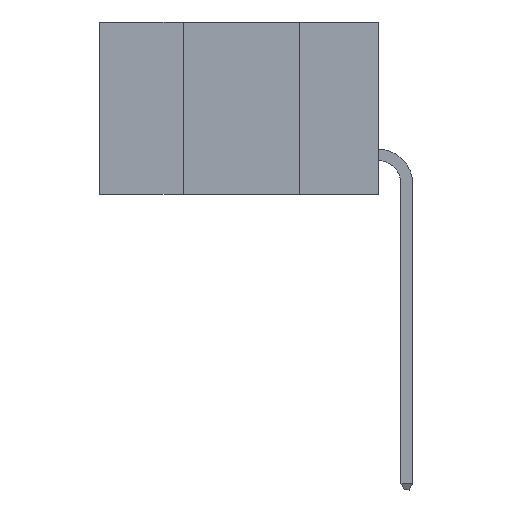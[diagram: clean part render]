
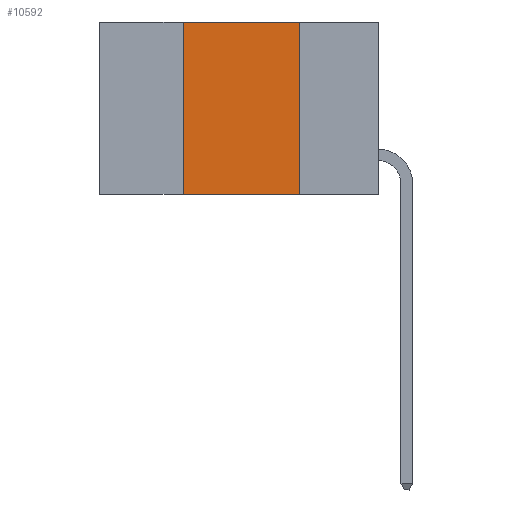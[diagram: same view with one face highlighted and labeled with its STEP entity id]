
A CAD part, left-side view. The second image highlights one B-rep face of the part: STEP entity #10592.
In plain terms, the highlighted planar face has unit normal (-1, 0, 0).
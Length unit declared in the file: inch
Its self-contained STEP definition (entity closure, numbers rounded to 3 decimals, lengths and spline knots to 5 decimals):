
#473 = CARTESIAN_POINT ( 'NONE',  ( 0., 0.42, 0. ) ) ;
#482 = CARTESIAN_POINT ( 'NONE',  ( 0., 0.17, -0.37 ) ) ;
#729 = VERTEX_POINT ( 'NONE', #4284 ) ;
#1281 = EDGE_CURVE ( 'NONE', #11646, #4821, #4223, .T. ) ;
#1575 = ORIENTED_EDGE ( 'NONE', *, *, #9898, .F. ) ;
#1997 = CARTESIAN_POINT ( 'NONE',  ( 0., 0.42, -0.37 ) ) ;
#2478 = LINE ( 'NONE', #9122, #4818 ) ;
#2542 = CARTESIAN_POINT ( 'NONE',  ( 0., 0.6, 0. ) ) ;
#2613 = LINE ( 'NONE', #4099, #10349 ) ;
#3326 = VECTOR ( 'NONE', #12554, 39.37008 ) ;
#3593 = DIRECTION ( 'NONE',  ( 1., 0., 0. ) ) ;
#4085 = CARTESIAN_POINT ( 'NONE',  ( 0., 0.42, 0. ) ) ;
#4093 = DIRECTION ( 'NONE',  ( 0., 0., -1. ) ) ;
#4099 = CARTESIAN_POINT ( 'NONE',  ( 0., 0.6, 0. ) ) ;
#4137 = DIRECTION ( 'NONE',  ( 0., -1., 0. ) ) ;
#4223 = LINE ( 'NONE', #5103, #12580 ) ;
#4284 = CARTESIAN_POINT ( 'NONE',  ( 0., 0.17, 0. ) ) ;
#4818 = VECTOR ( 'NONE', #4093, 39.37008 ) ;
#4821 = VERTEX_POINT ( 'NONE', #482 ) ;
#5103 = CARTESIAN_POINT ( 'NONE',  ( 0., 0.6, -0.37 ) ) ;
#5286 = VERTEX_POINT ( 'NONE', #4085 ) ;
#5787 = ORIENTED_EDGE ( 'NONE', *, *, #10683, .F. ) ;
#6057 = FACE_OUTER_BOUND ( 'NONE', #6111, .T. ) ;
#6111 = EDGE_LOOP ( 'NONE', ( #1575, #5787, #10129, #12408 ) ) ;
#6491 = PLANE ( 'NONE',  #11300 ) ;
#7238 = EDGE_CURVE ( 'NONE', #11646, #5286, #8992, .T. ) ;
#8992 = LINE ( 'NONE', #473, #3326 ) ;
#9122 = CARTESIAN_POINT ( 'NONE',  ( 0., 0.17, 0. ) ) ;
#9455 = DIRECTION ( 'NONE',  ( 0., 0., -1. ) ) ;
#9898 = EDGE_CURVE ( 'NONE', #729, #4821, #2478, .T. ) ;
#10129 = ORIENTED_EDGE ( 'NONE', *, *, #7238, .F. ) ;
#10349 = VECTOR ( 'NONE', #11756, 39.37008 ) ;
#10592 = ADVANCED_FACE ( 'NONE', ( #6057 ), #6491, .F. ) ;
#10683 = EDGE_CURVE ( 'NONE', #5286, #729, #2613, .T. ) ;
#11300 = AXIS2_PLACEMENT_3D ( 'NONE', #2542, #3593, #9455 ) ;
#11646 = VERTEX_POINT ( 'NONE', #1997 ) ;
#11756 = DIRECTION ( 'NONE',  ( 0., -1., 0. ) ) ;
#12408 = ORIENTED_EDGE ( 'NONE', *, *, #1281, .T. ) ;
#12554 = DIRECTION ( 'NONE',  ( 0., 0., 1. ) ) ;
#12580 = VECTOR ( 'NONE', #4137, 39.37008 ) ;
